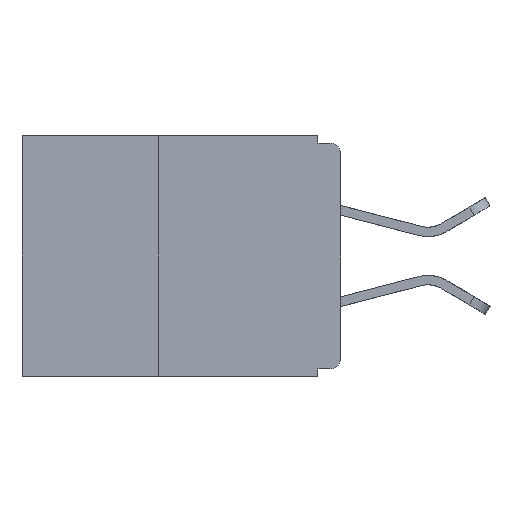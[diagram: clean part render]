
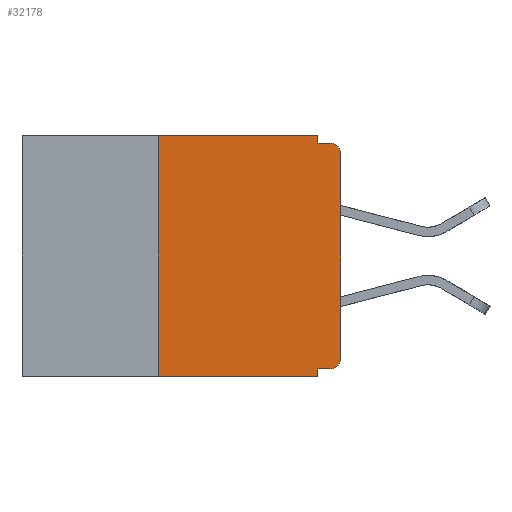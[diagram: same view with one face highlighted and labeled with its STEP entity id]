
A CAD part, left-side view. The second image highlights one B-rep face of the part: STEP entity #32178.
In plain terms, the highlighted planar face has unit normal (-1, 0, 0).
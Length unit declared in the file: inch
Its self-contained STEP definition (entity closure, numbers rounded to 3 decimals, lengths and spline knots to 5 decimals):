
#221 = CIRCLE ( 'NONE', #22090, 0.015 ) ;
#297 = ORIENTED_EDGE ( 'NONE', *, *, #12161, .F. ) ;
#580 = VECTOR ( 'NONE', #24734, 39.37008 ) ;
#845 = DIRECTION ( 'NONE',  ( 0., 1., 0. ) ) ;
#1013 = VERTEX_POINT ( 'NONE', #22653 ) ;
#1091 = LINE ( 'NONE', #13932, #6702 ) ;
#2045 = ORIENTED_EDGE ( 'NONE', *, *, #17176, .F. ) ;
#2351 = CIRCLE ( 'NONE', #23131, 0.015 ) ;
#2409 = VERTEX_POINT ( 'NONE', #4587 ) ;
#4017 = CARTESIAN_POINT ( 'NONE',  ( 0., 0.015, -0.025 ) ) ;
#4201 = ORIENTED_EDGE ( 'NONE', *, *, #14131, .T. ) ;
#4375 = FACE_OUTER_BOUND ( 'NONE', #13770, .T. ) ;
#4587 = CARTESIAN_POINT ( 'NONE',  ( 0., 0.031, -0.33 ) ) ;
#5449 = DIRECTION ( 'NONE',  ( 0., 0., -1. ) ) ;
#6363 = DIRECTION ( 'NONE',  ( -1., 0., 0. ) ) ;
#6702 = VECTOR ( 'NONE', #8569, 39.37008 ) ;
#6712 = VERTEX_POINT ( 'NONE', #13204 ) ;
#6814 = DIRECTION ( 'NONE',  ( 0., 0., -1. ) ) ;
#6892 = VECTOR ( 'NONE', #32303, 39.37008 ) ;
#7654 = ORIENTED_EDGE ( 'NONE', *, *, #23508, .T. ) ;
#7916 = LINE ( 'NONE', #29944, #580 ) ;
#8140 = CARTESIAN_POINT ( 'NONE',  ( 0., 0.437, 0. ) ) ;
#8456 = EDGE_CURVE ( 'NONE', #1013, #20873, #33718, .T. ) ;
#8569 = DIRECTION ( 'NONE',  ( 0., 0., -1. ) ) ;
#8789 = DIRECTION ( 'NONE',  ( 0., -1., 0. ) ) ;
#9002 = CARTESIAN_POINT ( 'NONE',  ( 0., 0., -0.32 ) ) ;
#9122 = CARTESIAN_POINT ( 'NONE',  ( 0., 0.25, -0.33 ) ) ;
#9996 = CARTESIAN_POINT ( 'NONE',  ( 0., 0., -0.01 ) ) ;
#10346 = LINE ( 'NONE', #9002, #28973 ) ;
#10499 = VECTOR ( 'NONE', #33737, 39.37008 ) ;
#11008 = DIRECTION ( 'NONE',  ( 0., -1., 0. ) ) ;
#11324 = VERTEX_POINT ( 'NONE', #9122 ) ;
#12161 = EDGE_CURVE ( 'NONE', #11324, #1013, #7916, .T. ) ;
#12612 = CARTESIAN_POINT ( 'NONE',  ( 0., 0., 0. ) ) ;
#13077 = ORIENTED_EDGE ( 'NONE', *, *, #13927, .F. ) ;
#13138 = EDGE_CURVE ( 'NONE', #15646, #32821, #25407, .T. ) ;
#13204 = CARTESIAN_POINT ( 'NONE',  ( 0., 0.031, -0.32 ) ) ;
#13445 = CARTESIAN_POINT ( 'NONE',  ( 0., 0., -0.305 ) ) ;
#13505 = EDGE_CURVE ( 'NONE', #32368, #34008, #221, .T. ) ;
#13770 = EDGE_LOOP ( 'NONE', ( #31628, #4201, #33251, #13077, #13909, #297, #7654, #2045, #16407, #23400 ) ) ;
#13909 = ORIENTED_EDGE ( 'NONE', *, *, #8456, .F. ) ;
#13927 = EDGE_CURVE ( 'NONE', #20873, #15646, #1091, .T. ) ;
#13932 = CARTESIAN_POINT ( 'NONE',  ( 0., 0.031, 0. ) ) ;
#14131 = EDGE_CURVE ( 'NONE', #24422, #32821, #2351, .T. ) ;
#14264 = EDGE_CURVE ( 'NONE', #34008, #24422, #17101, .T. ) ;
#15646 = VERTEX_POINT ( 'NONE', #28177 ) ;
#16407 = ORIENTED_EDGE ( 'NONE', *, *, #27717, .F. ) ;
#16916 = CARTESIAN_POINT ( 'NONE',  ( 0., 0.015, -0.32 ) ) ;
#17101 = LINE ( 'NONE', #12612, #19553 ) ;
#17176 = EDGE_CURVE ( 'NONE', #6712, #2409, #28023, .T. ) ;
#19553 = VECTOR ( 'NONE', #28450, 39.37008 ) ;
#20873 = VERTEX_POINT ( 'NONE', #28174 ) ;
#21412 = DIRECTION ( 'NONE',  ( 1., 0., 0. ) ) ;
#21424 = VECTOR ( 'NONE', #8789, 39.37008 ) ;
#21693 = CARTESIAN_POINT ( 'NONE',  ( 0., 0.437, -0.33 ) ) ;
#22090 = AXIS2_PLACEMENT_3D ( 'NONE', #22263, #6363, #24879 ) ;
#22263 = CARTESIAN_POINT ( 'NONE',  ( 0., 0.015, -0.305 ) ) ;
#22653 = CARTESIAN_POINT ( 'NONE',  ( 0., 0.25, 0. ) ) ;
#22690 = DIRECTION ( 'NONE',  ( -1., 0., 0. ) ) ;
#23131 = AXIS2_PLACEMENT_3D ( 'NONE', #4017, #22690, #6814 ) ;
#23400 = ORIENTED_EDGE ( 'NONE', *, *, #13505, .T. ) ;
#23508 = EDGE_CURVE ( 'NONE', #11324, #2409, #25068, .T. ) ;
#23522 = AXIS2_PLACEMENT_3D ( 'NONE', #26592, #21412, #5449 ) ;
#24222 = VECTOR ( 'NONE', #11008, 39.37008 ) ;
#24422 = VERTEX_POINT ( 'NONE', #28212 ) ;
#24445 = CARTESIAN_POINT ( 'NONE',  ( 0., 0.015, -0.01 ) ) ;
#24734 = DIRECTION ( 'NONE',  ( 0., 0., 1. ) ) ;
#24879 = DIRECTION ( 'NONE',  ( 0., 0., -1. ) ) ;
#25068 = LINE ( 'NONE', #21693, #24222 ) ;
#25407 = LINE ( 'NONE', #9996, #10499 ) ;
#26592 = CARTESIAN_POINT ( 'NONE',  ( 0., 0.437, 0. ) ) ;
#27717 = EDGE_CURVE ( 'NONE', #32368, #6712, #10346, .T. ) ;
#28023 = LINE ( 'NONE', #29690, #6892 ) ;
#28174 = CARTESIAN_POINT ( 'NONE',  ( 0., 0.031, 0. ) ) ;
#28177 = CARTESIAN_POINT ( 'NONE',  ( 0., 0.031, -0.01 ) ) ;
#28212 = CARTESIAN_POINT ( 'NONE',  ( 0., 0., -0.025 ) ) ;
#28450 = DIRECTION ( 'NONE',  ( 0., 0., 1. ) ) ;
#28973 = VECTOR ( 'NONE', #845, 39.37008 ) ;
#29690 = CARTESIAN_POINT ( 'NONE',  ( 0., 0.031, -0.33 ) ) ;
#29944 = CARTESIAN_POINT ( 'NONE',  ( 0., 0.25, -0.33 ) ) ;
#31628 = ORIENTED_EDGE ( 'NONE', *, *, #14264, .T. ) ;
#31863 = PLANE ( 'NONE',  #23522 ) ;
#32178 = ADVANCED_FACE ( 'NONE', ( #4375 ), #31863, .F. ) ;
#32303 = DIRECTION ( 'NONE',  ( 0., 0., -1. ) ) ;
#32368 = VERTEX_POINT ( 'NONE', #16916 ) ;
#32821 = VERTEX_POINT ( 'NONE', #24445 ) ;
#33251 = ORIENTED_EDGE ( 'NONE', *, *, #13138, .F. ) ;
#33718 = LINE ( 'NONE', #8140, #21424 ) ;
#33737 = DIRECTION ( 'NONE',  ( 0., -1., 0. ) ) ;
#34008 = VERTEX_POINT ( 'NONE', #13445 ) ;
